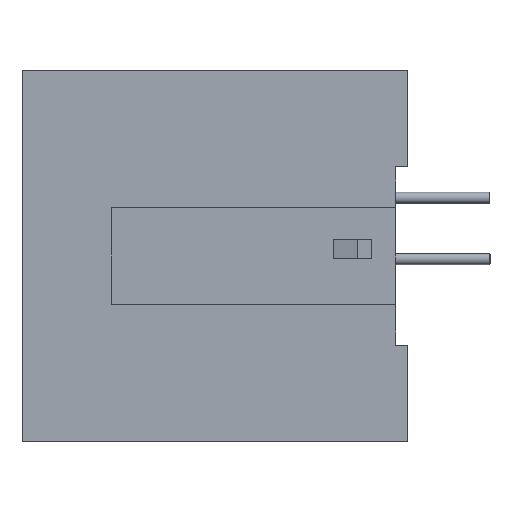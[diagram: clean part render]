
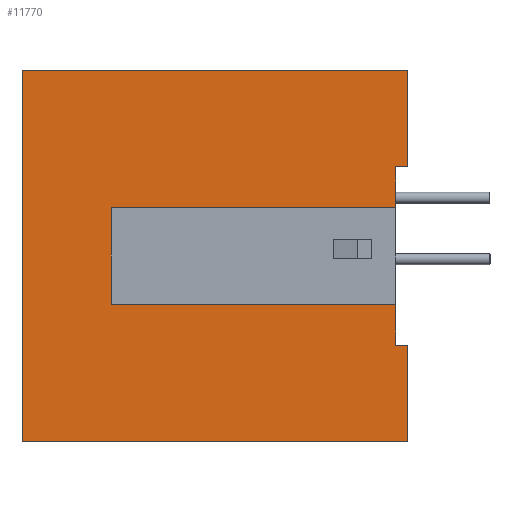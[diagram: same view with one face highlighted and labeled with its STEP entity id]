
A CAD part, left-side view. The second image highlights one B-rep face of the part: STEP entity #11770.
In plain terms, the highlighted planar face has unit normal (-1, 0, 0).
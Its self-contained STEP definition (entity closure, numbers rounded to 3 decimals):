
#44 = EDGE_LOOP ( 'NONE', ( #4889, #1128, #11800, #8621, #10253, #13547, #4565, #3564, #368, #13360, #4880, #5762 ) ) ;
#267 = LINE ( 'NONE', #7915, #13056 ) ;
#292 = CARTESIAN_POINT ( 'NONE',  ( -27.5, -7.8, 1.8 ) ) ;
#368 = ORIENTED_EDGE ( 'NONE', *, *, #9667, .F. ) ;
#428 = EDGE_CURVE ( 'NONE', #13604, #2377, #2614, .T. ) ;
#732 = CARTESIAN_POINT ( 'NONE',  ( -27.5, -8.3, 0. ) ) ;
#810 = DIRECTION ( 'NONE',  ( 0., 1., 0. ) ) ;
#811 = VERTEX_POINT ( 'NONE', #12527 ) ;
#907 = DIRECTION ( 'NONE',  ( 1., 0., 0. ) ) ;
#927 = DIRECTION ( 'NONE',  ( 0., 0., 1. ) ) ;
#963 = EDGE_CURVE ( 'NONE', #11134, #13604, #10532, .T. ) ;
#1115 = PLANE ( 'NONE',  #12139 ) ;
#1128 = ORIENTED_EDGE ( 'NONE', *, *, #8844, .T. ) ;
#1592 = DIRECTION ( 'NONE',  ( 0., 1., 0. ) ) ;
#1691 = VERTEX_POINT ( 'NONE', #9198 ) ;
#1712 = EDGE_CURVE ( 'NONE', #12049, #12647, #2677, .T. ) ;
#1823 = VECTOR ( 'NONE', #2807, 1000. ) ;
#1970 = VECTOR ( 'NONE', #1592, 1000. ) ;
#2003 = EDGE_CURVE ( 'NONE', #6570, #811, #6517, .T. ) ;
#2227 = CARTESIAN_POINT ( 'NONE',  ( -27.5, 4., -1.8 ) ) ;
#2377 = VERTEX_POINT ( 'NONE', #11793 ) ;
#2596 = CARTESIAN_POINT ( 'NONE',  ( -27.5, -8.3, 0. ) ) ;
#2614 = LINE ( 'NONE', #5893, #1970 ) ;
#2664 = VERTEX_POINT ( 'NONE', #5127 ) ;
#2677 = LINE ( 'NONE', #5037, #11022 ) ;
#2807 = DIRECTION ( 'NONE',  ( 0., 0., -1. ) ) ;
#2871 = DIRECTION ( 'NONE',  ( 0., 0., -1. ) ) ;
#3195 = FACE_OUTER_BOUND ( 'NONE', #44, .T. ) ;
#3378 = VERTEX_POINT ( 'NONE', #13741 ) ;
#3564 = ORIENTED_EDGE ( 'NONE', *, *, #7502, .F. ) ;
#3831 = VECTOR ( 'NONE', #810, 1000. ) ;
#3944 = VERTEX_POINT ( 'NONE', #10255 ) ;
#4484 = CARTESIAN_POINT ( 'NONE',  ( -27.5, -0.3, -3.7 ) ) ;
#4565 = ORIENTED_EDGE ( 'NONE', *, *, #1712, .F. ) ;
#4880 = ORIENTED_EDGE ( 'NONE', *, *, #963, .F. ) ;
#4889 = ORIENTED_EDGE ( 'NONE', *, *, #9564, .F. ) ;
#5037 = CARTESIAN_POINT ( 'NONE',  ( -27.5, -7.8, 0. ) ) ;
#5127 = CARTESIAN_POINT ( 'NONE',  ( -27.5, -8.3, -3.7 ) ) ;
#5179 = CARTESIAN_POINT ( 'NONE',  ( -27.5, -0.3, -7.7 ) ) ;
#5241 = CARTESIAN_POINT ( 'NONE',  ( -27.5, -7.8, 0. ) ) ;
#5280 = VECTOR ( 'NONE', #13874, 1000. ) ;
#5324 = DIRECTION ( 'NONE',  ( 0., 1., 0. ) ) ;
#5762 = ORIENTED_EDGE ( 'NONE', *, *, #8214, .F. ) ;
#5893 = CARTESIAN_POINT ( 'NONE',  ( -27.5, -0.3, 1.8 ) ) ;
#5945 = LINE ( 'NONE', #2596, #6344 ) ;
#6336 = VECTOR ( 'NONE', #5324, 1000. ) ;
#6344 = VECTOR ( 'NONE', #6801, 1000. ) ;
#6517 = LINE ( 'NONE', #5179, #3831 ) ;
#6570 = VERTEX_POINT ( 'NONE', #11221 ) ;
#6792 = CARTESIAN_POINT ( 'NONE',  ( -27.5, -7.8, 3.7 ) ) ;
#6801 = DIRECTION ( 'NONE',  ( 0., 0., -1. ) ) ;
#7028 = DIRECTION ( 'NONE',  ( 0., 0., -1. ) ) ;
#7477 = EDGE_CURVE ( 'NONE', #811, #3378, #13655, .T. ) ;
#7502 = EDGE_CURVE ( 'NONE', #10960, #12049, #9597, .T. ) ;
#7555 = DIRECTION ( 'NONE',  ( 0., 1., 0. ) ) ;
#7902 = VECTOR ( 'NONE', #2871, 1000. ) ;
#7915 = CARTESIAN_POINT ( 'NONE',  ( -27.5, -0.3, 3.7 ) ) ;
#7998 = EDGE_CURVE ( 'NONE', #12647, #2664, #12212, .T. ) ;
#8214 = EDGE_CURVE ( 'NONE', #1691, #11134, #267, .T. ) ;
#8329 = CARTESIAN_POINT ( 'NONE',  ( -27.5, -7.8, -1.8 ) ) ;
#8442 = CARTESIAN_POINT ( 'NONE',  ( -27.5, -0.3, -1.8 ) ) ;
#8453 = DIRECTION ( 'NONE',  ( 0., 0., -1. ) ) ;
#8529 = CARTESIAN_POINT ( 'NONE',  ( -27.5, 4., 0. ) ) ;
#8621 = ORIENTED_EDGE ( 'NONE', *, *, #2003, .F. ) ;
#8844 = EDGE_CURVE ( 'NONE', #3944, #3378, #14107, .T. ) ;
#9198 = CARTESIAN_POINT ( 'NONE',  ( -27.5, -8.3, 3.7 ) ) ;
#9310 = LINE ( 'NONE', #8529, #12289 ) ;
#9564 = EDGE_CURVE ( 'NONE', #3944, #1691, #5945, .T. ) ;
#9597 = LINE ( 'NONE', #8442, #5280 ) ;
#9667 = EDGE_CURVE ( 'NONE', #2377, #10960, #9310, .T. ) ;
#10253 = ORIENTED_EDGE ( 'NONE', *, *, #12591, .F. ) ;
#10255 = CARTESIAN_POINT ( 'NONE',  ( -27.5, -8.3, 7.7 ) ) ;
#10532 = LINE ( 'NONE', #5241, #7902 ) ;
#10852 = CARTESIAN_POINT ( 'NONE',  ( -27.5, -8.62, -8.008 ) ) ;
#10956 = CARTESIAN_POINT ( 'NONE',  ( -27.5, -0.3, 7.7 ) ) ;
#10960 = VERTEX_POINT ( 'NONE', #2227 ) ;
#11022 = VECTOR ( 'NONE', #7028, 1000. ) ;
#11134 = VERTEX_POINT ( 'NONE', #6792 ) ;
#11221 = CARTESIAN_POINT ( 'NONE',  ( -27.5, -8.3, -7.7 ) ) ;
#11770 = ADVANCED_FACE ( 'NONE', ( #3195 ), #1115, .F. ) ;
#11793 = CARTESIAN_POINT ( 'NONE',  ( -27.5, 4., 1.8 ) ) ;
#11800 = ORIENTED_EDGE ( 'NONE', *, *, #7477, .F. ) ;
#12049 = VERTEX_POINT ( 'NONE', #8329 ) ;
#12139 = AXIS2_PLACEMENT_3D ( 'NONE', #10852, #907, #7555 ) ;
#12212 = LINE ( 'NONE', #4484, #13965 ) ;
#12281 = DIRECTION ( 'NONE',  ( 0., 1., 0. ) ) ;
#12289 = VECTOR ( 'NONE', #8453, 1000. ) ;
#12527 = CARTESIAN_POINT ( 'NONE',  ( -27.5, 7.7, -7.7 ) ) ;
#12591 = EDGE_CURVE ( 'NONE', #2664, #6570, #12606, .T. ) ;
#12606 = LINE ( 'NONE', #732, #1823 ) ;
#12647 = VERTEX_POINT ( 'NONE', #12825 ) ;
#12825 = CARTESIAN_POINT ( 'NONE',  ( -27.5, -7.8, -3.7 ) ) ;
#13056 = VECTOR ( 'NONE', #12281, 1000. ) ;
#13146 = DIRECTION ( 'NONE',  ( 0., -1., 0. ) ) ;
#13266 = VECTOR ( 'NONE', #927, 1000. ) ;
#13360 = ORIENTED_EDGE ( 'NONE', *, *, #428, .F. ) ;
#13547 = ORIENTED_EDGE ( 'NONE', *, *, #7998, .F. ) ;
#13604 = VERTEX_POINT ( 'NONE', #292 ) ;
#13655 = LINE ( 'NONE', #14088, #13266 ) ;
#13741 = CARTESIAN_POINT ( 'NONE',  ( -27.5, 7.7, 7.7 ) ) ;
#13874 = DIRECTION ( 'NONE',  ( 0., -1., 0. ) ) ;
#13965 = VECTOR ( 'NONE', #13146, 1000. ) ;
#14088 = CARTESIAN_POINT ( 'NONE',  ( -27.5, 7.7, 0. ) ) ;
#14107 = LINE ( 'NONE', #10956, #6336 ) ;
